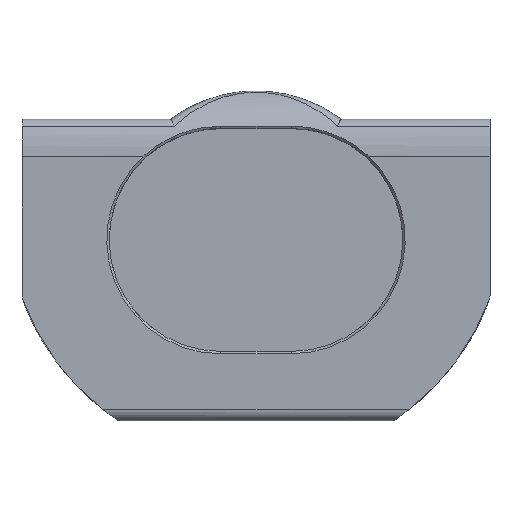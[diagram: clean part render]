
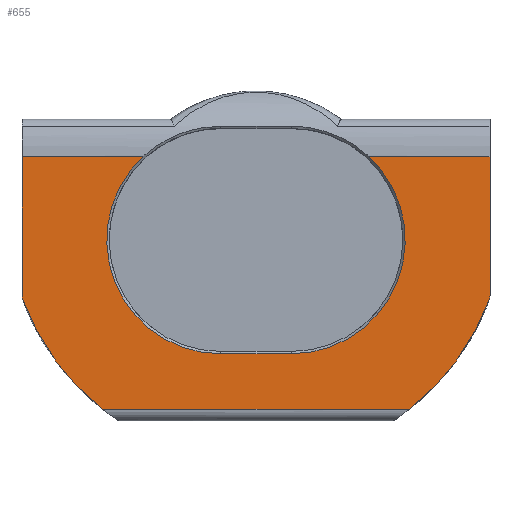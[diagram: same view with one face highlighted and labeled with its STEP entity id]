
A CAD part, top view. The second image highlights one B-rep face of the part: STEP entity #655.
In plain terms, the highlighted planar face has unit normal (0, 0, 1).
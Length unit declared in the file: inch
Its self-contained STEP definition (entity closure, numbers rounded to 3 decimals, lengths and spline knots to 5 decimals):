
#19=PLANE('',#718);
#36=CIRCLE('',#709,0.19458);
#37=CIRCLE('',#711,0.19458);
#40=CIRCLE('',#719,0.02);
#41=CIRCLE('',#720,0.425);
#42=CIRCLE('',#721,0.425);
#43=CIRCLE('',#722,0.02);
#60=LINE('',#1103,#108);
#72=LINE('',#1240,#120);
#73=LINE('',#1242,#121);
#74=LINE('',#1248,#122);
#75=LINE('',#1254,#123);
#76=LINE('',#1255,#124);
#108=VECTOR('',#802,0.3937);
#120=VECTOR('',#824,0.3937);
#121=VECTOR('',#825,0.3937);
#122=VECTOR('',#830,0.3937);
#123=VECTOR('',#835,0.3937);
#124=VECTOR('',#836,0.3937);
#186=FACE_OUTER_BOUND('',#224,.T.);
#224=EDGE_LOOP('',(#500,#501,#502,#503,#504,#505,#506,#507,#508,#509,#510,
#511));
#286=VERTEX_POINT('',#1085);
#289=VERTEX_POINT('',#1090);
#291=VERTEX_POINT('',#1095);
#292=VERTEX_POINT('',#1097);
#305=VERTEX_POINT('',#1239);
#306=VERTEX_POINT('',#1241);
#307=VERTEX_POINT('',#1243);
#308=VERTEX_POINT('',#1245);
#309=VERTEX_POINT('',#1247);
#310=VERTEX_POINT('',#1249);
#311=VERTEX_POINT('',#1251);
#312=VERTEX_POINT('',#1253);
#356=EDGE_CURVE('',#289,#286,#36,.T.);
#358=EDGE_CURVE('',#291,#292,#37,.T.);
#361=EDGE_CURVE('',#292,#289,#60,.T.);
#382=EDGE_CURVE('',#305,#291,#72,.T.);
#383=EDGE_CURVE('',#306,#305,#73,.T.);
#384=EDGE_CURVE('',#307,#306,#40,.T.);
#385=EDGE_CURVE('',#307,#308,#41,.T.);
#386=EDGE_CURVE('',#309,#308,#74,.T.);
#387=EDGE_CURVE('',#309,#310,#42,.T.);
#388=EDGE_CURVE('',#311,#310,#43,.T.);
#389=EDGE_CURVE('',#312,#311,#75,.T.);
#390=EDGE_CURVE('',#286,#312,#76,.T.);
#500=ORIENTED_EDGE('',*,*,#356,.F.);
#501=ORIENTED_EDGE('',*,*,#361,.F.);
#502=ORIENTED_EDGE('',*,*,#358,.F.);
#503=ORIENTED_EDGE('',*,*,#382,.F.);
#504=ORIENTED_EDGE('',*,*,#383,.F.);
#505=ORIENTED_EDGE('',*,*,#384,.F.);
#506=ORIENTED_EDGE('',*,*,#385,.T.);
#507=ORIENTED_EDGE('',*,*,#386,.F.);
#508=ORIENTED_EDGE('',*,*,#387,.T.);
#509=ORIENTED_EDGE('',*,*,#388,.F.);
#510=ORIENTED_EDGE('',*,*,#389,.F.);
#511=ORIENTED_EDGE('',*,*,#390,.F.);
#655=ADVANCED_FACE('',(#186),#19,.F.);
#709=AXIS2_PLACEMENT_3D('',#1092,#790,#791);
#711=AXIS2_PLACEMENT_3D('',#1098,#795,#796);
#718=AXIS2_PLACEMENT_3D('',#1238,#822,#823);
#719=AXIS2_PLACEMENT_3D('',#1244,#826,#827);
#720=AXIS2_PLACEMENT_3D('',#1246,#828,#829);
#721=AXIS2_PLACEMENT_3D('',#1250,#831,#832);
#722=AXIS2_PLACEMENT_3D('',#1252,#833,#834);
#790=DIRECTION('center_axis',(0.,0.,1.));
#791=DIRECTION('ref_axis',(0.,-1.,0.));
#795=DIRECTION('center_axis',(0.,0.,1.));
#796=DIRECTION('ref_axis',(-1.,0.,0.));
#802=DIRECTION('',(1.,0.,0.));
#822=DIRECTION('center_axis',(0.,0.,-1.));
#823=DIRECTION('ref_axis',(0.,-1.,0.));
#824=DIRECTION('',(1.,0.,0.));
#825=DIRECTION('',(0.,1.,0.));
#826=DIRECTION('center_axis',(0.,0.,-1.));
#827=DIRECTION('ref_axis',(-0.984,-0.176,0.));
#828=DIRECTION('center_axis',(0.,0.,1.));
#829=DIRECTION('ref_axis',(0.972,0.233,0.));
#830=DIRECTION('',(-1.,0.,0.));
#831=DIRECTION('center_axis',(0.,0.,1.));
#832=DIRECTION('ref_axis',(0.972,0.233,0.));
#833=DIRECTION('center_axis',(0.,0.,-1.));
#834=DIRECTION('ref_axis',(0.984,-0.176,0.));
#835=DIRECTION('',(0.,-1.,0.));
#836=DIRECTION('',(1.,0.,0.));
#1085=CARTESIAN_POINT('',(-0.25445,0.66667,-0.12792));
#1090=CARTESIAN_POINT('',(-0.38715,0.32977,-0.12792));
#1092=CARTESIAN_POINT('Origin',(-0.38715,0.52435,-0.12792));
#1095=CARTESIAN_POINT('',(-0.64084,0.66667,-0.12792));
#1097=CARTESIAN_POINT('',(-0.50815,0.32977,-0.12792));
#1098=CARTESIAN_POINT('Origin',(-0.50815,0.52435,-0.12792));
#1103=CARTESIAN_POINT('',(-0.2174,0.32977,-0.12792));
#1238=CARTESIAN_POINT('Origin',(-0.04765,0.84108,-0.12792));
#1239=CARTESIAN_POINT('',(-0.84765,0.66667,-0.12792));
#1240=CARTESIAN_POINT('',(-0.04765,0.66667,-0.12792));
#1241=CARTESIAN_POINT('',(-0.84765,0.42926,-0.12792));
#1242=CARTESIAN_POINT('',(-0.84765,0.42054,-0.12792));
#1243=CARTESIAN_POINT('',(-0.84641,0.42234,-0.12792));
#1244=CARTESIAN_POINT('Origin',(-0.82765,0.42926,-0.12792));
#1245=CARTESIAN_POINT('',(-0.70988,0.2349,-0.12792));
#1246=CARTESIAN_POINT('Origin',(-0.44765,0.56935,-0.12792));
#1247=CARTESIAN_POINT('',(-0.18542,0.2349,-0.12792));
#1248=CARTESIAN_POINT('',(-0.04765,0.2349,-0.12792));
#1249=CARTESIAN_POINT('',(-0.04888,0.42234,-0.12792));
#1250=CARTESIAN_POINT('Origin',(-0.44765,0.56935,-0.12792));
#1251=CARTESIAN_POINT('',(-0.04765,0.42926,-0.12792));
#1252=CARTESIAN_POINT('Origin',(-0.06765,0.42926,-0.12792));
#1253=CARTESIAN_POINT('',(-0.04765,0.66667,-0.12792));
#1254=CARTESIAN_POINT('',(-0.04765,0.42054,-0.12792));
#1255=CARTESIAN_POINT('',(-0.04765,0.66667,-0.12792));
